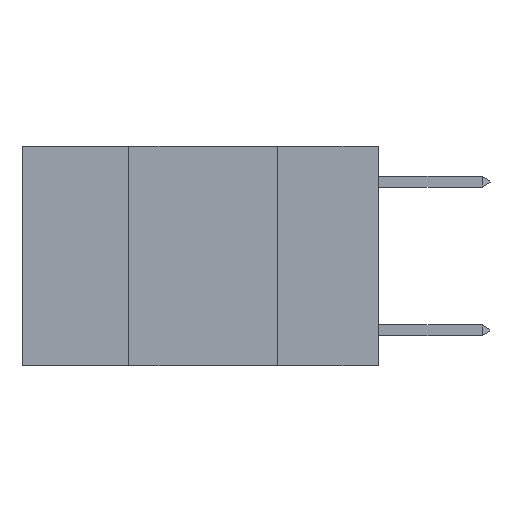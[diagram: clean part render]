
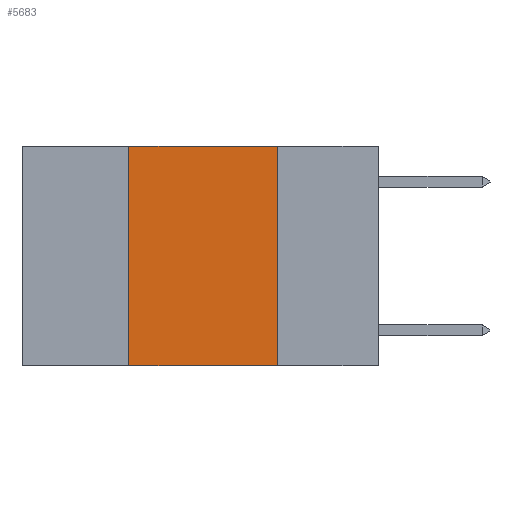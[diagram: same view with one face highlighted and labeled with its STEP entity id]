
A CAD part, left-side view. The second image highlights one B-rep face of the part: STEP entity #5683.
In plain terms, the highlighted planar face has unit normal (-1, 0, 0).
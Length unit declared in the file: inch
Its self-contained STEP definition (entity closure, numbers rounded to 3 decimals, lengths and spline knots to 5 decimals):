
#152 = EDGE_CURVE ( 'NONE', #6544, #5232, #3599, .T. ) ;
#324 = ORIENTED_EDGE ( 'NONE', *, *, #8202, .F. ) ;
#402 = VECTOR ( 'NONE', #1415, 39.37008 ) ;
#766 = LINE ( 'NONE', #2170, #9428 ) ;
#869 = VECTOR ( 'NONE', #7786, 39.37008 ) ;
#997 = DIRECTION ( 'NONE',  ( 0., 0., -1. ) ) ;
#1008 = DIRECTION ( 'NONE',  ( 1., 0., 0. ) ) ;
#1415 = DIRECTION ( 'NONE',  ( 0., 0., -1. ) ) ;
#1456 = CARTESIAN_POINT ( 'NONE',  ( 0., 0.17, 0. ) ) ;
#1629 = LINE ( 'NONE', #6993, #869 ) ;
#1872 = DIRECTION ( 'NONE',  ( 0., 0., 1. ) ) ;
#2170 = CARTESIAN_POINT ( 'NONE',  ( 0., 0.6, 0. ) ) ;
#2522 = CARTESIAN_POINT ( 'NONE',  ( 0., 0.42, 0. ) ) ;
#3599 = LINE ( 'NONE', #4477, #3609 ) ;
#3609 = VECTOR ( 'NONE', #1872, 39.37008 ) ;
#4181 = VERTEX_POINT ( 'NONE', #8909 ) ;
#4477 = CARTESIAN_POINT ( 'NONE',  ( 0., 0.42, 0. ) ) ;
#4580 = ORIENTED_EDGE ( 'NONE', *, *, #152, .F. ) ;
#4748 = CARTESIAN_POINT ( 'NONE',  ( 0., 0.17, -0.37 ) ) ;
#5232 = VERTEX_POINT ( 'NONE', #2522 ) ;
#5619 = FACE_OUTER_BOUND ( 'NONE', #8560, .T. ) ;
#5683 = ADVANCED_FACE ( 'NONE', ( #5619 ), #7507, .F. ) ;
#6414 = ORIENTED_EDGE ( 'NONE', *, *, #9242, .F. ) ;
#6544 = VERTEX_POINT ( 'NONE', #8604 ) ;
#6962 = LINE ( 'NONE', #1456, #402 ) ;
#6993 = CARTESIAN_POINT ( 'NONE',  ( 0., 0.6, -0.37 ) ) ;
#7085 = ORIENTED_EDGE ( 'NONE', *, *, #10298, .T. ) ;
#7126 = CARTESIAN_POINT ( 'NONE',  ( 0., 0.6, 0. ) ) ;
#7507 = PLANE ( 'NONE',  #8969 ) ;
#7763 = VERTEX_POINT ( 'NONE', #4748 ) ;
#7786 = DIRECTION ( 'NONE',  ( 0., -1., 0. ) ) ;
#7873 = DIRECTION ( 'NONE',  ( 0., -1., 0. ) ) ;
#8202 = EDGE_CURVE ( 'NONE', #4181, #7763, #6962, .T. ) ;
#8560 = EDGE_LOOP ( 'NONE', ( #324, #6414, #4580, #7085 ) ) ;
#8604 = CARTESIAN_POINT ( 'NONE',  ( 0., 0.42, -0.37 ) ) ;
#8909 = CARTESIAN_POINT ( 'NONE',  ( 0., 0.17, 0. ) ) ;
#8969 = AXIS2_PLACEMENT_3D ( 'NONE', #7126, #1008, #997 ) ;
#9242 = EDGE_CURVE ( 'NONE', #5232, #4181, #766, .T. ) ;
#9428 = VECTOR ( 'NONE', #7873, 39.37008 ) ;
#10298 = EDGE_CURVE ( 'NONE', #6544, #7763, #1629, .T. ) ;
